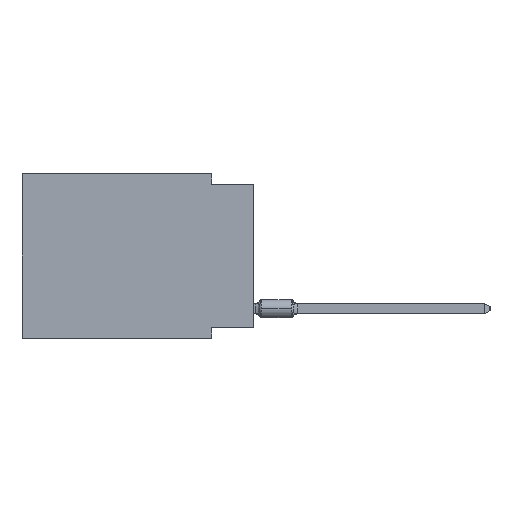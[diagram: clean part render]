
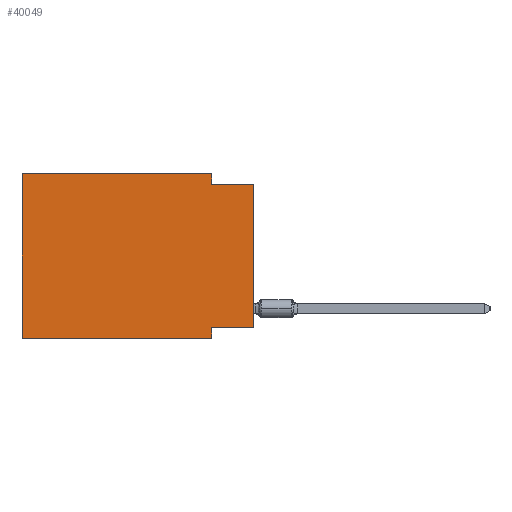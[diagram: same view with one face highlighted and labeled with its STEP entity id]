
A CAD part, left-side view. The second image highlights one B-rep face of the part: STEP entity #40049.
In plain terms, the highlighted planar face has unit normal (-1, 0, 0).
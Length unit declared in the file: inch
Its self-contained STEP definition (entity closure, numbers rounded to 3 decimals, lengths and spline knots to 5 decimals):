
#81 = LINE ( 'NONE', #10705, #18853 ) ;
#365 = CARTESIAN_POINT ( 'NONE',  ( 0., 0.55, -0.39 ) ) ;
#1017 = VERTEX_POINT ( 'NONE', #12888 ) ;
#1321 = DIRECTION ( 'NONE',  ( 0., 0., 1. ) ) ;
#2239 = DIRECTION ( 'NONE',  ( 0., 0., 1. ) ) ;
#2658 = FACE_OUTER_BOUND ( 'NONE', #21142, .T. ) ;
#2769 = ORIENTED_EDGE ( 'NONE', *, *, #2783, .T. ) ;
#2783 = EDGE_CURVE ( 'NONE', #40290, #21189, #17810, .T. ) ;
#3538 = DIRECTION ( 'NONE',  ( 0., 0., -1. ) ) ;
#3622 = VECTOR ( 'NONE', #18877, 39.37008 ) ;
#4086 = LINE ( 'NONE', #11025, #41541 ) ;
#4873 = EDGE_CURVE ( 'NONE', #6304, #5495, #38916, .T. ) ;
#4940 = DIRECTION ( 'NONE',  ( 0., 0., -1. ) ) ;
#5145 = VERTEX_POINT ( 'NONE', #13933 ) ;
#5495 = VERTEX_POINT ( 'NONE', #32748 ) ;
#5708 = EDGE_CURVE ( 'NONE', #6304, #38546, #16415, .T. ) ;
#6199 = ORIENTED_EDGE ( 'NONE', *, *, #4873, .F. ) ;
#6304 = VERTEX_POINT ( 'NONE', #40900 ) ;
#7316 = DIRECTION ( 'NONE',  ( 0., -1., 0. ) ) ;
#7694 = VECTOR ( 'NONE', #34927, 39.37008 ) ;
#8888 = ORIENTED_EDGE ( 'NONE', *, *, #5708, .T. ) ;
#9140 = CARTESIAN_POINT ( 'NONE',  ( 0., 0.55, 0. ) ) ;
#10477 = LINE ( 'NONE', #23689, #12544 ) ;
#10705 = CARTESIAN_POINT ( 'NONE',  ( 0., 0.1, -0.39 ) ) ;
#11025 = CARTESIAN_POINT ( 'NONE',  ( 0., 0.1, 0. ) ) ;
#12544 = VECTOR ( 'NONE', #20230, 39.37008 ) ;
#12840 = DIRECTION ( 'NONE',  ( 1., 0., 0. ) ) ;
#12888 = CARTESIAN_POINT ( 'NONE',  ( 0., 0.1, -0.025 ) ) ;
#13757 = CARTESIAN_POINT ( 'NONE',  ( 0., 0., -0.365 ) ) ;
#13933 = CARTESIAN_POINT ( 'NONE',  ( 0., 0.1, -0.365 ) ) ;
#15700 = AXIS2_PLACEMENT_3D ( 'NONE', #23241, #12840, #33214 ) ;
#16415 = LINE ( 'NONE', #365, #31657 ) ;
#17215 = CARTESIAN_POINT ( 'NONE',  ( 0., 0.1, -0.39 ) ) ;
#17810 = LINE ( 'NONE', #31032, #18959 ) ;
#18853 = VECTOR ( 'NONE', #3538, 39.37008 ) ;
#18877 = DIRECTION ( 'NONE',  ( 0., -1., 0. ) ) ;
#18959 = VECTOR ( 'NONE', #1321, 39.37008 ) ;
#19155 = EDGE_CURVE ( 'NONE', #1017, #21189, #30821, .T. ) ;
#19981 = PLANE ( 'NONE',  #15700 ) ;
#20153 = ORIENTED_EDGE ( 'NONE', *, *, #19155, .F. ) ;
#20230 = DIRECTION ( 'NONE',  ( 0., 1., 0. ) ) ;
#20393 = ORIENTED_EDGE ( 'NONE', *, *, #27822, .F. ) ;
#20496 = ORIENTED_EDGE ( 'NONE', *, *, #32888, .F. ) ;
#21142 = EDGE_LOOP ( 'NONE', ( #2769, #20153, #20393, #20496, #6199, #8888, #38413, #38160 ) ) ;
#21189 = VERTEX_POINT ( 'NONE', #32022 ) ;
#23241 = CARTESIAN_POINT ( 'NONE',  ( 0., 0.55, 0. ) ) ;
#23689 = CARTESIAN_POINT ( 'NONE',  ( 0., 0., -0.365 ) ) ;
#26476 = VERTEX_POINT ( 'NONE', #39050 ) ;
#27546 = CARTESIAN_POINT ( 'NONE',  ( 0., 0., -0.025 ) ) ;
#27822 = EDGE_CURVE ( 'NONE', #26476, #1017, #4086, .T. ) ;
#29995 = EDGE_CURVE ( 'NONE', #40290, #5145, #10477, .T. ) ;
#30821 = LINE ( 'NONE', #27546, #7694 ) ;
#31032 = CARTESIAN_POINT ( 'NONE',  ( 0., 0., 0. ) ) ;
#31255 = EDGE_CURVE ( 'NONE', #5145, #38546, #81, .T. ) ;
#31657 = VECTOR ( 'NONE', #7316, 39.37008 ) ;
#31947 = CARTESIAN_POINT ( 'NONE',  ( 0., 0.55, 0. ) ) ;
#32022 = CARTESIAN_POINT ( 'NONE',  ( 0., 0., -0.025 ) ) ;
#32748 = CARTESIAN_POINT ( 'NONE',  ( 0., 0.55, 0. ) ) ;
#32888 = EDGE_CURVE ( 'NONE', #5495, #26476, #35798, .T. ) ;
#33214 = DIRECTION ( 'NONE',  ( 0., 0., -1. ) ) ;
#34927 = DIRECTION ( 'NONE',  ( 0., -1., 0. ) ) ;
#35798 = LINE ( 'NONE', #9140, #3622 ) ;
#35821 = VECTOR ( 'NONE', #2239, 39.37008 ) ;
#38160 = ORIENTED_EDGE ( 'NONE', *, *, #29995, .F. ) ;
#38413 = ORIENTED_EDGE ( 'NONE', *, *, #31255, .F. ) ;
#38546 = VERTEX_POINT ( 'NONE', #17215 ) ;
#38916 = LINE ( 'NONE', #31947, #35821 ) ;
#39050 = CARTESIAN_POINT ( 'NONE',  ( 0., 0.1, 0. ) ) ;
#40049 = ADVANCED_FACE ( 'NONE', ( #2658 ), #19981, .F. ) ;
#40290 = VERTEX_POINT ( 'NONE', #13757 ) ;
#40900 = CARTESIAN_POINT ( 'NONE',  ( 0., 0.55, -0.39 ) ) ;
#41541 = VECTOR ( 'NONE', #4940, 39.37008 ) ;
